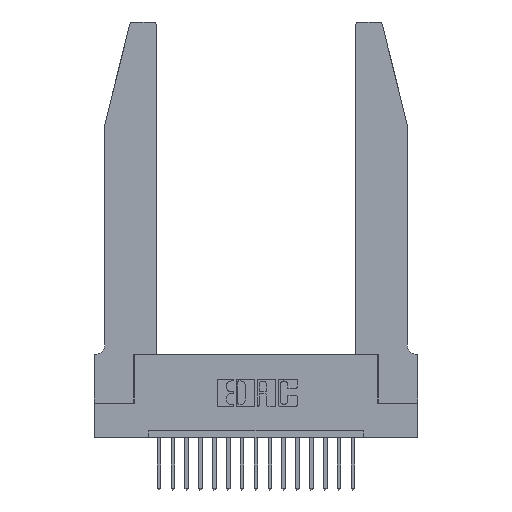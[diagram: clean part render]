
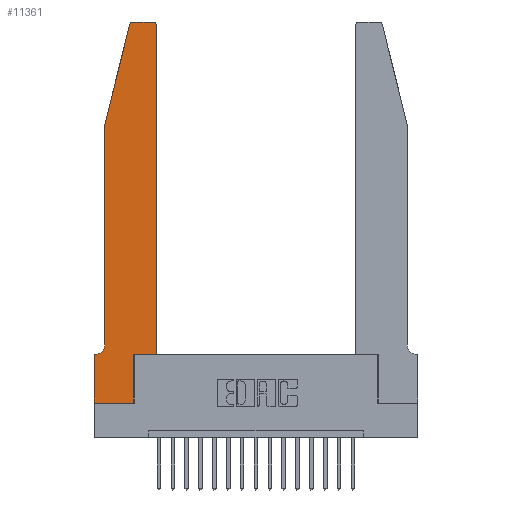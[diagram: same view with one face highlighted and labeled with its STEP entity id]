
A CAD part, top view. The second image highlights one B-rep face of the part: STEP entity #11361.
In plain terms, the highlighted planar face has unit normal (0, 0, 1).
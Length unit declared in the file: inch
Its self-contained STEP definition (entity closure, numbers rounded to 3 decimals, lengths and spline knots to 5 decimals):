
#24 = DIRECTION ( 'NONE',  ( 0., 0., 1. ) ) ;
#82 = EDGE_CURVE ( 'NONE', #890, #10078, #9998, .T. ) ;
#214 = CARTESIAN_POINT ( 'NONE',  ( 0.284, 2.75, 0.37 ) ) ;
#277 = DIRECTION ( 'NONE',  ( 0., -1., 0. ) ) ;
#351 = EDGE_CURVE ( 'NONE', #12721, #1376, #11869, .T. ) ;
#465 = DIRECTION ( 'NONE',  ( -1., 0., 0. ) ) ;
#748 = ORIENTED_EDGE ( 'NONE', *, *, #2994, .T. ) ;
#890 = VERTEX_POINT ( 'NONE', #12495 ) ;
#907 = DIRECTION ( 'NONE',  ( -1., 0., 0. ) ) ;
#1017 = CARTESIAN_POINT ( 'NONE',  ( 0.2865, 0.35, 0.37 ) ) ;
#1106 = VECTOR ( 'NONE', #465, 39.37008 ) ;
#1249 = CARTESIAN_POINT ( 'NONE',  ( 0., 0., 0.37 ) ) ;
#1336 = LINE ( 'NONE', #17076, #1106 ) ;
#1376 = VERTEX_POINT ( 'NONE', #11650 ) ;
#1508 = DIRECTION ( 'NONE',  ( 0., 1., 0. ) ) ;
#1555 = VERTEX_POINT ( 'NONE', #3062 ) ;
#1562 = CARTESIAN_POINT ( 'NONE',  ( 0.4505, 0.35, 0.37 ) ) ;
#1966 = CARTESIAN_POINT ( 'NONE',  ( 0.0755, 2., 0.37 ) ) ;
#2120 = ORIENTED_EDGE ( 'NONE', *, *, #82, .T. ) ;
#2144 = EDGE_CURVE ( 'NONE', #13698, #17069, #17080, .T. ) ;
#2162 = EDGE_CURVE ( 'NONE', #11463, #13172, #1336, .T. ) ;
#2347 = VECTOR ( 'NONE', #1508, 39.37008 ) ;
#2994 = EDGE_CURVE ( 'NONE', #10078, #17435, #17272, .T. ) ;
#3062 = CARTESIAN_POINT ( 'NONE',  ( 0.0055, 0.35, 0.37 ) ) ;
#3183 = PLANE ( 'NONE',  #7108 ) ;
#4300 = ORIENTED_EDGE ( 'NONE', *, *, #6261, .T. ) ;
#5300 = CARTESIAN_POINT ( 'NONE',  ( 0.4505, 0.35, 0.37 ) ) ;
#5320 = AXIS2_PLACEMENT_3D ( 'NONE', #13564, #8722, #13302 ) ;
#5873 = CARTESIAN_POINT ( 'NONE',  ( 0., 0.35, 0.37 ) ) ;
#5950 = VECTOR ( 'NONE', #11842, 39.37008 ) ;
#5990 = VECTOR ( 'NONE', #6154, 39.37008 ) ;
#6154 = DIRECTION ( 'NONE',  ( 1., 0., 0. ) ) ;
#6261 = EDGE_CURVE ( 'NONE', #13172, #13740, #9533, .T. ) ;
#6304 = CARTESIAN_POINT ( 'NONE',  ( 0., 0.35, 0.37 ) ) ;
#6334 = AXIS2_PLACEMENT_3D ( 'NONE', #11551, #11803, #907 ) ;
#6410 = LINE ( 'NONE', #13744, #12999 ) ;
#6444 = CARTESIAN_POINT ( 'NONE',  ( 0.4205, 2.75, 0.37 ) ) ;
#6478 = LINE ( 'NONE', #1562, #5990 ) ;
#6654 = DIRECTION ( 'NONE',  ( 0., 1., 0. ) ) ;
#6913 = CARTESIAN_POINT ( 'NONE',  ( 0.25487, 2.72718, 0.37 ) ) ;
#7054 = ORIENTED_EDGE ( 'NONE', *, *, #10092, .T. ) ;
#7108 = AXIS2_PLACEMENT_3D ( 'NONE', #6304, #24, #12174 ) ;
#7279 = ORIENTED_EDGE ( 'NONE', *, *, #12926, .T. ) ;
#7564 = VECTOR ( 'NONE', #6654, 39.37008 ) ;
#7842 = LINE ( 'NONE', #1249, #9949 ) ;
#7965 = DIRECTION ( 'NONE',  ( -1., 0., 0. ) ) ;
#8085 = CARTESIAN_POINT ( 'NONE',  ( 0.2865, 0.35, 0.37 ) ) ;
#8542 = ORIENTED_EDGE ( 'NONE', *, *, #13065, .T. ) ;
#8647 = CIRCLE ( 'NONE', #6334, 0.07 ) ;
#8722 = DIRECTION ( 'NONE',  ( 0., 0., 1. ) ) ;
#9049 = VECTOR ( 'NONE', #16279, 39.37008 ) ;
#9117 = VERTEX_POINT ( 'NONE', #5873 ) ;
#9533 = CIRCLE ( 'NONE', #16294, 0.03 ) ;
#9949 = VECTOR ( 'NONE', #18028, 39.37008 ) ;
#9998 = LINE ( 'NONE', #19092, #9049 ) ;
#10078 = VERTEX_POINT ( 'NONE', #15640 ) ;
#10092 = EDGE_CURVE ( 'NONE', #17069, #1555, #8647, .T. ) ;
#10111 = CARTESIAN_POINT ( 'NONE',  ( 0.4505, 0.35, 0.37 ) ) ;
#10306 = CARTESIAN_POINT ( 'NONE',  ( 0.0755, 2., 0.37 ) ) ;
#11243 = ORIENTED_EDGE ( 'NONE', *, *, #2144, .T. ) ;
#11361 = ADVANCED_FACE ( 'NONE', ( #13351 ), #3183, .T. ) ;
#11463 = VERTEX_POINT ( 'NONE', #6444 ) ;
#11551 = CARTESIAN_POINT ( 'NONE',  ( 0.0055, 0.42, 0.37 ) ) ;
#11590 = CARTESIAN_POINT ( 'NONE',  ( 0.284, 2.72, 0.37 ) ) ;
#11650 = CARTESIAN_POINT ( 'NONE',  ( 0.4505, 2.72, 0.37 ) ) ;
#11803 = DIRECTION ( 'NONE',  ( 0., 0., -1. ) ) ;
#11842 = DIRECTION ( 'NONE',  ( -0.239, -0.971, 0. ) ) ;
#11869 = LINE ( 'NONE', #10111, #2347 ) ;
#11940 = CARTESIAN_POINT ( 'NONE',  ( 0.0755, 0.42, 0.37 ) ) ;
#12174 = DIRECTION ( 'NONE',  ( 1., 0., 0. ) ) ;
#12495 = CARTESIAN_POINT ( 'NONE',  ( 0., 0., 0.37 ) ) ;
#12539 = VECTOR ( 'NONE', #277, 39.37008 ) ;
#12721 = VERTEX_POINT ( 'NONE', #5300 ) ;
#12842 = EDGE_CURVE ( 'NONE', #9117, #890, #7842, .T. ) ;
#12926 = EDGE_CURVE ( 'NONE', #1376, #11463, #17326, .T. ) ;
#12999 = VECTOR ( 'NONE', #7965, 39.37008 ) ;
#13065 = EDGE_CURVE ( 'NONE', #13740, #13698, #15424, .T. ) ;
#13140 = CARTESIAN_POINT ( 'NONE',  ( 0.0755, 2., 0.37 ) ) ;
#13172 = VERTEX_POINT ( 'NONE', #214 ) ;
#13302 = DIRECTION ( 'NONE',  ( 1., 0., 0. ) ) ;
#13351 = FACE_OUTER_BOUND ( 'NONE', #17833, .T. ) ;
#13363 = ORIENTED_EDGE ( 'NONE', *, *, #2162, .T. ) ;
#13564 = CARTESIAN_POINT ( 'NONE',  ( 0.4205, 2.72, 0.37 ) ) ;
#13698 = VERTEX_POINT ( 'NONE', #13140 ) ;
#13740 = VERTEX_POINT ( 'NONE', #6913 ) ;
#13744 = CARTESIAN_POINT ( 'NONE',  ( 0.0755, 0.35, 0.37 ) ) ;
#13797 = EDGE_CURVE ( 'NONE', #1555, #9117, #6410, .T. ) ;
#14556 = EDGE_CURVE ( 'NONE', #17435, #12721, #6478, .T. ) ;
#14852 = DIRECTION ( 'NONE',  ( 0., 0., 1. ) ) ;
#15424 = LINE ( 'NONE', #10306, #5950 ) ;
#15640 = CARTESIAN_POINT ( 'NONE',  ( 0.2865, 0., 0.37 ) ) ;
#15974 = ORIENTED_EDGE ( 'NONE', *, *, #351, .T. ) ;
#16279 = DIRECTION ( 'NONE',  ( 1., 0., 0. ) ) ;
#16294 = AXIS2_PLACEMENT_3D ( 'NONE', #11590, #14852, #17835 ) ;
#16606 = ORIENTED_EDGE ( 'NONE', *, *, #14556, .T. ) ;
#17069 = VERTEX_POINT ( 'NONE', #11940 ) ;
#17076 = CARTESIAN_POINT ( 'NONE',  ( 0.2605, 2.75, 0.37 ) ) ;
#17080 = LINE ( 'NONE', #1966, #12539 ) ;
#17272 = LINE ( 'NONE', #8085, #7564 ) ;
#17326 = CIRCLE ( 'NONE', #5320, 0.03 ) ;
#17435 = VERTEX_POINT ( 'NONE', #1017 ) ;
#17524 = ORIENTED_EDGE ( 'NONE', *, *, #12842, .T. ) ;
#17833 = EDGE_LOOP ( 'NONE', ( #13363, #4300, #8542, #11243, #7054, #18901, #17524, #2120, #748, #16606, #15974, #7279 ) ) ;
#17835 = DIRECTION ( 'NONE',  ( 1., 0., 0. ) ) ;
#18028 = DIRECTION ( 'NONE',  ( 0., -1., 0. ) ) ;
#18901 = ORIENTED_EDGE ( 'NONE', *, *, #13797, .T. ) ;
#19092 = CARTESIAN_POINT ( 'NONE',  ( 0., 0., 0.37 ) ) ;
